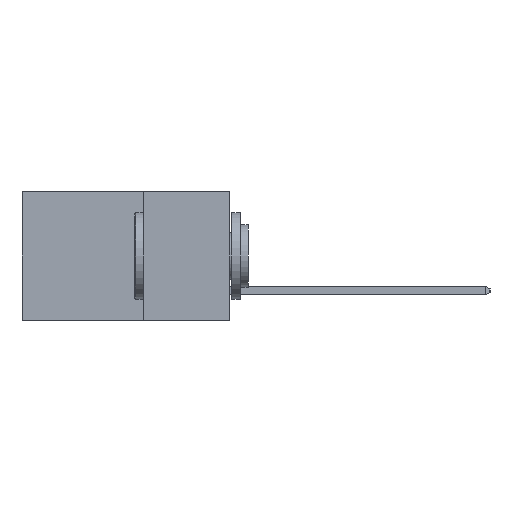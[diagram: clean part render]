
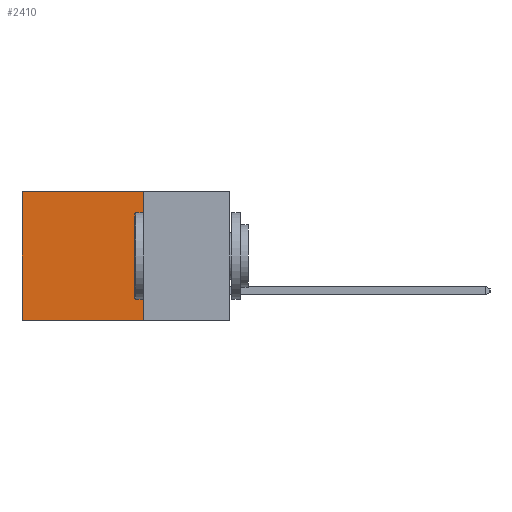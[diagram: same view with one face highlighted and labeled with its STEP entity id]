
A CAD part, left-side view. The second image highlights one B-rep face of the part: STEP entity #2410.
In plain terms, the highlighted planar face has unit normal (-1, 0, 0).
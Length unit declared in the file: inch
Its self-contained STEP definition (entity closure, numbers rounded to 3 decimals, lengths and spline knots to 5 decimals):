
#5 = CARTESIAN_POINT ( 'NONE',  ( 0.298, 0.6, 0. ) ) ;
#358 = EDGE_CURVE ( 'NONE', #6399, #3756, #7665, .T. ) ;
#423 = VECTOR ( 'NONE', #9165, 39.37008 ) ;
#750 = AXIS2_PLACEMENT_3D ( 'NONE', #6860, #5870, #10793 ) ;
#852 = LINE ( 'NONE', #9209, #423 ) ;
#1760 = EDGE_CURVE ( 'NONE', #3756, #3805, #13336, .T. ) ;
#2152 = VECTOR ( 'NONE', #13795, 39.37008 ) ;
#2410 = ADVANCED_FACE ( 'NONE', ( #15927 ), #9042, .F. ) ;
#3207 = DIRECTION ( 'NONE',  ( 0., 1., 0. ) ) ;
#3756 = VERTEX_POINT ( 'NONE', #8390 ) ;
#3805 = VERTEX_POINT ( 'NONE', #4410 ) ;
#4410 = CARTESIAN_POINT ( 'NONE',  ( 0.298, 0.6, -0.37 ) ) ;
#4577 = EDGE_CURVE ( 'NONE', #6399, #8704, #852, .T. ) ;
#4743 = CARTESIAN_POINT ( 'NONE',  ( 0.298, 0.25, 0. ) ) ;
#4845 = VECTOR ( 'NONE', #13286, 39.37008 ) ;
#5801 = LINE ( 'NONE', #9735, #2152 ) ;
#5870 = DIRECTION ( 'NONE',  ( 1., 0., 0. ) ) ;
#6399 = VERTEX_POINT ( 'NONE', #4743 ) ;
#6460 = EDGE_CURVE ( 'NONE', #8704, #3805, #5801, .T. ) ;
#6860 = CARTESIAN_POINT ( 'NONE',  ( 0.298, 0.25, 0. ) ) ;
#7307 = ORIENTED_EDGE ( 'NONE', *, *, #1760, .F. ) ;
#7665 = LINE ( 'NONE', #14043, #4845 ) ;
#8289 = CARTESIAN_POINT ( 'NONE',  ( 0.298, 0.25, -0.37 ) ) ;
#8390 = CARTESIAN_POINT ( 'NONE',  ( 0.298, 0.25, -0.37 ) ) ;
#8704 = VERTEX_POINT ( 'NONE', #5 ) ;
#8819 = ORIENTED_EDGE ( 'NONE', *, *, #358, .F. ) ;
#9042 = PLANE ( 'NONE',  #750 ) ;
#9165 = DIRECTION ( 'NONE',  ( 0., 1., 0. ) ) ;
#9209 = CARTESIAN_POINT ( 'NONE',  ( 0.298, 0.25, 0. ) ) ;
#9735 = CARTESIAN_POINT ( 'NONE',  ( 0.298, 0.6, 0. ) ) ;
#10101 = VECTOR ( 'NONE', #3207, 39.37008 ) ;
#10793 = DIRECTION ( 'NONE',  ( 0., 0., -1. ) ) ;
#10804 = ORIENTED_EDGE ( 'NONE', *, *, #6460, .T. ) ;
#13286 = DIRECTION ( 'NONE',  ( 0., 0., -1. ) ) ;
#13336 = LINE ( 'NONE', #8289, #10101 ) ;
#13795 = DIRECTION ( 'NONE',  ( 0., 0., -1. ) ) ;
#14043 = CARTESIAN_POINT ( 'NONE',  ( 0.298, 0.25, 0. ) ) ;
#14144 = EDGE_LOOP ( 'NONE', ( #10804, #7307, #8819, #14892 ) ) ;
#14892 = ORIENTED_EDGE ( 'NONE', *, *, #4577, .T. ) ;
#15927 = FACE_OUTER_BOUND ( 'NONE', #14144, .T. ) ;
